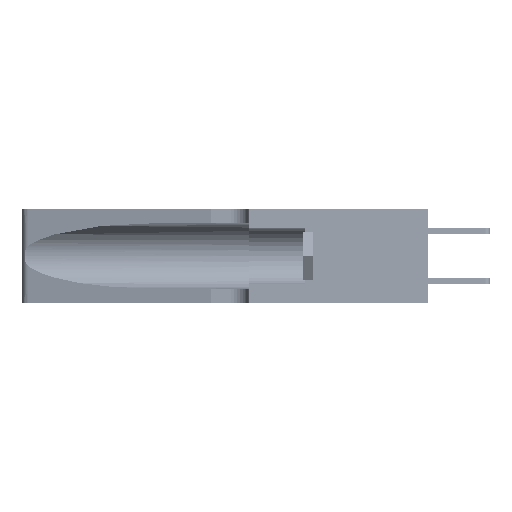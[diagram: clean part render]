
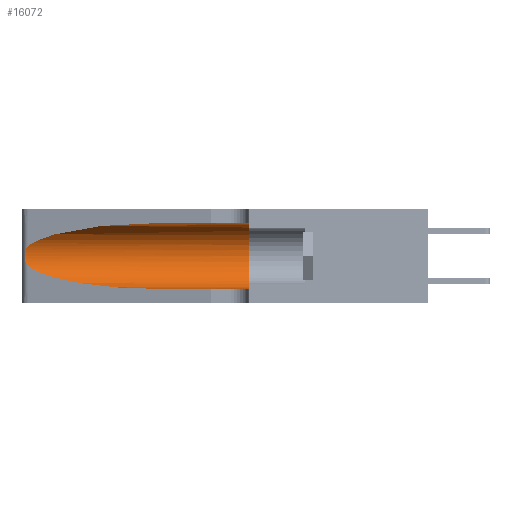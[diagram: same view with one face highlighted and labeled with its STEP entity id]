
A CAD part, left-side view. The second image highlights one B-rep face of the part: STEP entity #16072.
In plain terms, the highlighted cylindrical face has radius 3.308 mm (diameter 6.617 mm), a partial arc.
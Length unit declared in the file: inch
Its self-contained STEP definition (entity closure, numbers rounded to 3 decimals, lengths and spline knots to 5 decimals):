
#489 = CARTESIAN_POINT ( 'NONE',  ( 0.1305, 0.35, 0.185 ) ) ;
#1059 = DIRECTION ( 'NONE',  ( 0., -1., 0. ) ) ;
#1104 = CARTESIAN_POINT ( 'NONE',  ( 0.25487, 1.22718, 0.14631 ) ) ;
#1270 = CARTESIAN_POINT ( 'NONE',  ( 0.1305, 0.72297, 0.05475 ) ) ;
#1607 = CARTESIAN_POINT ( 'NONE',  ( 0.18966, 0.96281, 0.05475 ) ) ;
#1772 = CARTESIAN_POINT ( 'NONE',  ( 0.1305, 1.61858, 0.185 ) ) ;
#2425 = CARTESIAN_POINT ( 'NONE',  ( 0.26017, 1.23833, 0.17102 ) ) ;
#2585 = CARTESIAN_POINT ( 'NONE',  ( 0.25789, 1.23486, 0.15765 ) ) ;
#3046 = DIRECTION ( 'NONE',  ( 0., -1., 0. ) ) ;
#3606 = ORIENTED_EDGE ( 'NONE', *, *, #28077, .T. ) ;
#5224 = CARTESIAN_POINT ( 'NONE',  ( 0.2373, 1.15595, 0.08982 ) ) ;
#5573 = CYLINDRICAL_SURFACE ( 'NONE', #15348, 0.13025 ) ;
#5645 = ORIENTED_EDGE ( 'NONE', *, *, #11223, .T. ) ;
#6181 = CARTESIAN_POINT ( 'NONE',  ( 0.26018, 1.23835, 0.19895 ) ) ;
#6414 = ORIENTED_EDGE ( 'NONE', *, *, #24983, .T. ) ;
#9915 = CARTESIAN_POINT ( 'NONE',  ( 0.1305, 0.72297, 0.31525 ) ) ;
#11223 = EDGE_CURVE ( 'NONE', #34439, #26040, #49727, .T. ) ;
#11382 = EDGE_CURVE ( 'NONE', #44982, #18832, #48880, .T. ) ;
#11677 = DIRECTION ( 'NONE',  ( 0., 1., 0. ) ) ;
#14014 = VERTEX_POINT ( 'NONE', #24367 ) ;
#14193 = CARTESIAN_POINT ( 'NONE',  ( 0.18966, 0.96281, 0.31525 ) ) ;
#14233 = CARTESIAN_POINT ( 'NONE',  ( 0.26075, 1.23896, 0.19203 ) ) ;
#14339 = LINE ( 'NONE', #50620, #16832 ) ;
#15348 = AXIS2_PLACEMENT_3D ( 'NONE', #1772, #49106, #49270 ) ;
#16072 = ADVANCED_FACE ( 'NONE', ( #47941 ), #5573, .F. ) ;
#16832 = VECTOR ( 'NONE', #1059, 39.37008 ) ;
#18036 = CARTESIAN_POINT ( 'NONE',  ( 0.25639, 1.23186, 0.15144 ) ) ;
#18328 = EDGE_LOOP ( 'NONE', ( #5645, #6414, #3606, #33124, #47005, #32644 ) ) ;
#18660 = CARTESIAN_POINT ( 'NONE',  ( 0.1305, 1.61858, 0.05475 ) ) ;
#18832 = VERTEX_POINT ( 'NONE', #22738 ) ;
#19414 = EDGE_CURVE ( 'NONE', #23922, #18832, #45033, .T. ) ;
#21824 = CARTESIAN_POINT ( 'NONE',  ( 0.25555, 1.22994, 0.2215 ) ) ;
#22738 = CARTESIAN_POINT ( 'NONE',  ( 0.1305, 0.35, 0.05475 ) ) ;
#23922 = VERTEX_POINT ( 'NONE', #50340 ) ;
#24367 = CARTESIAN_POINT ( 'NONE',  ( 0.25487, 1.22718, 0.14631 ) ) ;
#24982 = AXIS2_PLACEMENT_3D ( 'NONE', #489, #11677, #35645 ) ;
#24983 = EDGE_CURVE ( 'NONE', #26040, #14014, #36787, .T. ) ;
#25749 = CARTESIAN_POINT ( 'NONE',  ( 0.25639, 1.23184, 0.21858 ) ) ;
#26040 = VERTEX_POINT ( 'NONE', #28222 ) ;
#27043 = CARTESIAN_POINT ( 'NONE',  ( 0.1305, 0.72297, 0.31525 ) ) ;
#27725 =( BOUNDED_CURVE ( )  B_SPLINE_CURVE ( 3, ( #1104, #5224, #1607, #1270 ),
 .UNSPECIFIED., .F., .T. ) 
 B_SPLINE_CURVE_WITH_KNOTS ( ( 4, 4 ),
 ( 3.44316, 4.71239 ),
 .UNSPECIFIED. ) 
 CURVE ( )  GEOMETRIC_REPRESENTATION_ITEM ( )  RATIONAL_B_SPLINE_CURVE ( ( 1., 0.87, 0.87, 1. ) ) 
 REPRESENTATION_ITEM ( '' )  );
#28077 = EDGE_CURVE ( 'NONE', #14014, #44982, #27725, .T. ) ;
#28222 = CARTESIAN_POINT ( 'NONE',  ( 0.25487, 1.22718, 0.22369 ) ) ;
#28365 = EDGE_CURVE ( 'NONE', #34439, #23922, #14339, .T. ) ;
#29871 = CARTESIAN_POINT ( 'NONE',  ( 0.25487, 1.22718, 0.22369 ) ) ;
#30476 = VECTOR ( 'NONE', #3046, 39.37008 ) ;
#32644 = ORIENTED_EDGE ( 'NONE', *, *, #28365, .F. ) ;
#33124 = ORIENTED_EDGE ( 'NONE', *, *, #11382, .T. ) ;
#33897 = CARTESIAN_POINT ( 'NONE',  ( 0.25487, 1.22718, 0.22369 ) ) ;
#34111 = CARTESIAN_POINT ( 'NONE',  ( 0.25854, 1.2359, 0.20912 ) ) ;
#34439 = VERTEX_POINT ( 'NONE', #27043 ) ;
#35645 = DIRECTION ( 'NONE',  ( 0., 0., 1. ) ) ;
#35961 = CARTESIAN_POINT ( 'NONE',  ( 0.1305, 0.72297, 0.05475 ) ) ;
#36787 = B_SPLINE_CURVE_WITH_KNOTS ( 'NONE', 3,
 ( #29871, #21824, #25749, #42023, #34111, #6181, #14233, #49582, #2425, #45969, #2585, #18036, #41520, #41851 ),
 .UNSPECIFIED., .F., .F.,
 ( 4, 2, 2, 2, 2, 2, 4 ),
 ( 0., 0.00027, 0.00053, 0.00107, 0.0016, 0.00187, 0.00214 ),
 .UNSPECIFIED. ) ;
#37498 = CARTESIAN_POINT ( 'NONE',  ( 0.2373, 1.15595, 0.28018 ) ) ;
#41520 = CARTESIAN_POINT ( 'NONE',  ( 0.25555, 1.22993, 0.14849 ) ) ;
#41851 = CARTESIAN_POINT ( 'NONE',  ( 0.25487, 1.22718, 0.14631 ) ) ;
#42023 = CARTESIAN_POINT ( 'NONE',  ( 0.25787, 1.23484, 0.2124 ) ) ;
#44982 = VERTEX_POINT ( 'NONE', #35961 ) ;
#45033 = CIRCLE ( 'NONE', #24982, 0.13025 ) ;
#45969 = CARTESIAN_POINT ( 'NONE',  ( 0.25856, 1.23593, 0.16098 ) ) ;
#47005 = ORIENTED_EDGE ( 'NONE', *, *, #19414, .F. ) ;
#47941 = FACE_OUTER_BOUND ( 'NONE', #18328, .T. ) ;
#48880 = LINE ( 'NONE', #18660, #30476 ) ;
#49106 = DIRECTION ( 'NONE',  ( 0., -1., 0. ) ) ;
#49270 = DIRECTION ( 'NONE',  ( 0., 0., -1. ) ) ;
#49582 = CARTESIAN_POINT ( 'NONE',  ( 0.26075, 1.23896, 0.178 ) ) ;
#49727 =( BOUNDED_CURVE ( )  B_SPLINE_CURVE ( 3, ( #9915, #14193, #37498, #33897 ),
 .UNSPECIFIED., .F., .F. ) 
 B_SPLINE_CURVE_WITH_KNOTS ( ( 4, 4 ),
 ( 1.5708, 2.84003 ),
 .UNSPECIFIED. ) 
 CURVE ( )  GEOMETRIC_REPRESENTATION_ITEM ( )  RATIONAL_B_SPLINE_CURVE ( ( 1., 0.87, 0.87, 1. ) ) 
 REPRESENTATION_ITEM ( '' )  );
#50340 = CARTESIAN_POINT ( 'NONE',  ( 0.1305, 0.35, 0.31525 ) ) ;
#50620 = CARTESIAN_POINT ( 'NONE',  ( 0.1305, 1.61858, 0.31525 ) ) ;
